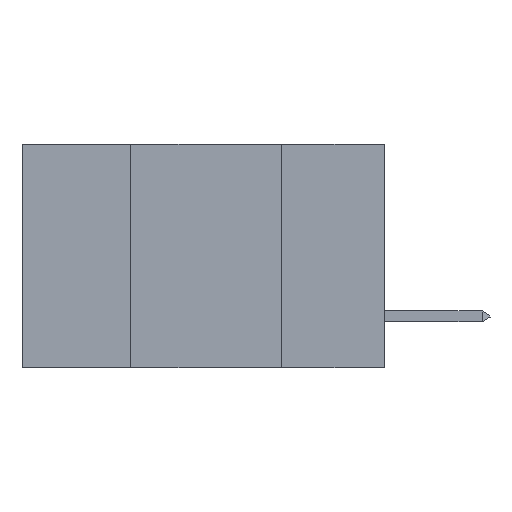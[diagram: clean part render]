
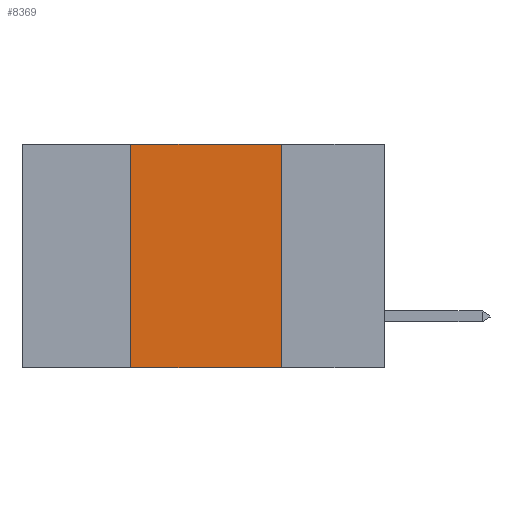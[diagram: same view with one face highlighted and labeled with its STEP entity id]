
A CAD part, left-side view. The second image highlights one B-rep face of the part: STEP entity #8369.
In plain terms, the highlighted planar face has unit normal (-1, 0, 0).
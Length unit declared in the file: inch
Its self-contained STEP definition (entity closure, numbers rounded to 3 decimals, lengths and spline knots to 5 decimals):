
#378 = EDGE_CURVE ( 'NONE', #12932, #8078, #9345, .T. ) ;
#449 = DIRECTION ( 'NONE',  ( 0., 0., -1. ) ) ;
#624 = EDGE_CURVE ( 'NONE', #12872, #12932, #5379, .T. ) ;
#680 = CARTESIAN_POINT ( 'NONE',  ( 0., 0.17, 0. ) ) ;
#1130 = FACE_OUTER_BOUND ( 'NONE', #1508, .T. ) ;
#1508 = EDGE_LOOP ( 'NONE', ( #13273, #11768, #9141, #2130 ) ) ;
#2130 = ORIENTED_EDGE ( 'NONE', *, *, #3419, .T. ) ;
#3263 = CARTESIAN_POINT ( 'NONE',  ( 0., 0.42, -0.37 ) ) ;
#3419 = EDGE_CURVE ( 'NONE', #12872, #7423, #12511, .T. ) ;
#3888 = CARTESIAN_POINT ( 'NONE',  ( 0., 0.17, -0.37 ) ) ;
#4000 = DIRECTION ( 'NONE',  ( 0., 0., -1. ) ) ;
#4214 = CARTESIAN_POINT ( 'NONE',  ( 0., 0.17, 0. ) ) ;
#4493 = CARTESIAN_POINT ( 'NONE',  ( 0., 0.6, 0. ) ) ;
#4588 = VECTOR ( 'NONE', #11009, 39.37008 ) ;
#4782 = DIRECTION ( 'NONE',  ( 0., -1., 0. ) ) ;
#4809 = LINE ( 'NONE', #680, #10845 ) ;
#5351 = EDGE_CURVE ( 'NONE', #8078, #7423, #4809, .T. ) ;
#5379 = LINE ( 'NONE', #6682, #13198 ) ;
#6682 = CARTESIAN_POINT ( 'NONE',  ( 0., 0.42, 0. ) ) ;
#6916 = VECTOR ( 'NONE', #4782, 39.37008 ) ;
#7423 = VERTEX_POINT ( 'NONE', #3888 ) ;
#7936 = CARTESIAN_POINT ( 'NONE',  ( 0., 0.6, -0.37 ) ) ;
#8078 = VERTEX_POINT ( 'NONE', #4214 ) ;
#8369 = ADVANCED_FACE ( 'NONE', ( #1130 ), #10707, .F. ) ;
#9141 = ORIENTED_EDGE ( 'NONE', *, *, #624, .F. ) ;
#9214 = AXIS2_PLACEMENT_3D ( 'NONE', #4493, #12714, #449 ) ;
#9345 = LINE ( 'NONE', #10084, #4588 ) ;
#9672 = DIRECTION ( 'NONE',  ( 0., 0., 1. ) ) ;
#10084 = CARTESIAN_POINT ( 'NONE',  ( 0., 0.6, 0. ) ) ;
#10707 = PLANE ( 'NONE',  #9214 ) ;
#10845 = VECTOR ( 'NONE', #4000, 39.37008 ) ;
#11009 = DIRECTION ( 'NONE',  ( 0., -1., 0. ) ) ;
#11768 = ORIENTED_EDGE ( 'NONE', *, *, #378, .F. ) ;
#12034 = CARTESIAN_POINT ( 'NONE',  ( 0., 0.42, 0. ) ) ;
#12511 = LINE ( 'NONE', #7936, #6916 ) ;
#12714 = DIRECTION ( 'NONE',  ( 1., 0., 0. ) ) ;
#12872 = VERTEX_POINT ( 'NONE', #3263 ) ;
#12932 = VERTEX_POINT ( 'NONE', #12034 ) ;
#13198 = VECTOR ( 'NONE', #9672, 39.37008 ) ;
#13273 = ORIENTED_EDGE ( 'NONE', *, *, #5351, .F. ) ;
